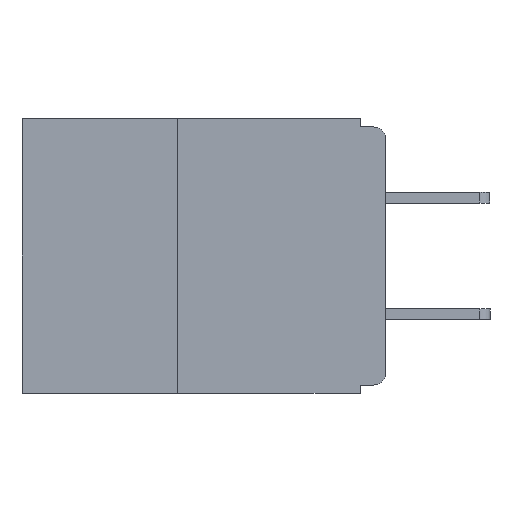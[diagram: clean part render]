
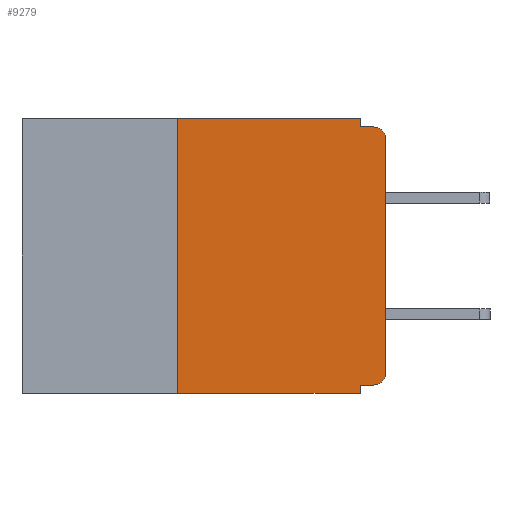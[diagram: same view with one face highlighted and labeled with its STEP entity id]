
A CAD part, left-side view. The second image highlights one B-rep face of the part: STEP entity #9279.
In plain terms, the highlighted planar face has unit normal (-1, 0, 0).
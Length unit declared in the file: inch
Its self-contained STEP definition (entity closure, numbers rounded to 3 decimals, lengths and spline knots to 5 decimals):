
#222 = CARTESIAN_POINT ( 'NONE',  ( 0., 0.25, -0.33 ) ) ;
#572 = DIRECTION ( 'NONE',  ( 0., -1., 0. ) ) ;
#774 = CARTESIAN_POINT ( 'NONE',  ( 0., 0., -0.01 ) ) ;
#980 = VECTOR ( 'NONE', #4086, 39.37008 ) ;
#1192 = DIRECTION ( 'NONE',  ( 0., 1., 0. ) ) ;
#1337 = LINE ( 'NONE', #5362, #1765 ) ;
#1546 = AXIS2_PLACEMENT_3D ( 'NONE', #6348, #11543, #3697 ) ;
#1620 = AXIS2_PLACEMENT_3D ( 'NONE', #16402, #16381, #16363 ) ;
#1765 = VECTOR ( 'NONE', #13138, 39.37008 ) ;
#1864 = DIRECTION ( 'NONE',  ( -1., 0., 0. ) ) ;
#1917 = CARTESIAN_POINT ( 'NONE',  ( 0., 0.25, 0. ) ) ;
#2356 = EDGE_CURVE ( 'NONE', #12118, #11571, #12422, .T. ) ;
#2382 = VECTOR ( 'NONE', #11886, 39.37008 ) ;
#2617 = VERTEX_POINT ( 'NONE', #5564 ) ;
#3012 = EDGE_CURVE ( 'NONE', #12989, #3067, #9993, .T. ) ;
#3044 = VECTOR ( 'NONE', #572, 39.37008 ) ;
#3067 = VERTEX_POINT ( 'NONE', #11272 ) ;
#3249 = CARTESIAN_POINT ( 'NONE',  ( 0., 0.25, -0.33 ) ) ;
#3310 = ORIENTED_EDGE ( 'NONE', *, *, #14291, .T. ) ;
#3428 = DIRECTION ( 'NONE',  ( 0., 0., 1. ) ) ;
#3697 = DIRECTION ( 'NONE',  ( 0., 0., -1. ) ) ;
#3735 = ORIENTED_EDGE ( 'NONE', *, *, #9853, .T. ) ;
#3780 = ORIENTED_EDGE ( 'NONE', *, *, #7662, .F. ) ;
#3961 = ORIENTED_EDGE ( 'NONE', *, *, #3012, .T. ) ;
#3988 = DIRECTION ( 'NONE',  ( 0., 0., -1. ) ) ;
#4086 = DIRECTION ( 'NONE',  ( 0., 0., -1. ) ) ;
#4179 = ORIENTED_EDGE ( 'NONE', *, *, #16122, .F. ) ;
#5362 = CARTESIAN_POINT ( 'NONE',  ( 0., 0.437, 0. ) ) ;
#5399 = CARTESIAN_POINT ( 'NONE',  ( 0., 0.015, -0.32 ) ) ;
#5564 = CARTESIAN_POINT ( 'NONE',  ( 0., 0.031, 0. ) ) ;
#6177 = EDGE_CURVE ( 'NONE', #16425, #6324, #16328, .T. ) ;
#6249 = EDGE_CURVE ( 'NONE', #6316, #6324, #11846, .T. ) ;
#6273 = CARTESIAN_POINT ( 'NONE',  ( 0., 0.031, -0.32 ) ) ;
#6316 = VERTEX_POINT ( 'NONE', #15924 ) ;
#6324 = VERTEX_POINT ( 'NONE', #15846 ) ;
#6348 = CARTESIAN_POINT ( 'NONE',  ( 0., 0.437, 0. ) ) ;
#6741 = CARTESIAN_POINT ( 'NONE',  ( 0., 0.031, 0. ) ) ;
#7026 = VECTOR ( 'NONE', #1192, 39.37008 ) ;
#7049 = LINE ( 'NONE', #11306, #16777 ) ;
#7131 = VECTOR ( 'NONE', #3428, 39.37008 ) ;
#7381 = DIRECTION ( 'NONE',  ( 0., -1., 0. ) ) ;
#7662 = EDGE_CURVE ( 'NONE', #13566, #9763, #13954, .T. ) ;
#7985 = CARTESIAN_POINT ( 'NONE',  ( 0., 0., 0. ) ) ;
#8919 = PLANE ( 'NONE',  #1546 ) ;
#9279 = ADVANCED_FACE ( 'NONE', ( #13320 ), #8919, .F. ) ;
#9763 = VERTEX_POINT ( 'NONE', #1917 ) ;
#9853 = EDGE_CURVE ( 'NONE', #13566, #11571, #7049, .T. ) ;
#9993 = CIRCLE ( 'NONE', #15067, 0.015 ) ;
#10115 = ORIENTED_EDGE ( 'NONE', *, *, #14780, .F. ) ;
#10314 = ORIENTED_EDGE ( 'NONE', *, *, #6177, .F. ) ;
#10717 = EDGE_CURVE ( 'NONE', #2617, #16425, #11516, .T. ) ;
#11117 = ORIENTED_EDGE ( 'NONE', *, *, #10717, .F. ) ;
#11272 = CARTESIAN_POINT ( 'NONE',  ( 0., 0., -0.305 ) ) ;
#11306 = CARTESIAN_POINT ( 'NONE',  ( 0., 0.437, -0.33 ) ) ;
#11322 = VECTOR ( 'NONE', #14431, 39.37008 ) ;
#11516 = LINE ( 'NONE', #6741, #980 ) ;
#11543 = DIRECTION ( 'NONE',  ( 1., 0., 0. ) ) ;
#11571 = VERTEX_POINT ( 'NONE', #16553 ) ;
#11846 = CIRCLE ( 'NONE', #1620, 0.015 ) ;
#11886 = DIRECTION ( 'NONE',  ( 0., 0., -1. ) ) ;
#12118 = VERTEX_POINT ( 'NONE', #6273 ) ;
#12422 = LINE ( 'NONE', #14348, #2382 ) ;
#12748 = CARTESIAN_POINT ( 'NONE',  ( 0., 0.031, -0.01 ) ) ;
#12855 = CARTESIAN_POINT ( 'NONE',  ( 0., 0.015, -0.305 ) ) ;
#12989 = VERTEX_POINT ( 'NONE', #5399 ) ;
#13138 = DIRECTION ( 'NONE',  ( 0., -1., 0. ) ) ;
#13320 = FACE_OUTER_BOUND ( 'NONE', #15656, .T. ) ;
#13502 = ORIENTED_EDGE ( 'NONE', *, *, #2356, .F. ) ;
#13566 = VERTEX_POINT ( 'NONE', #222 ) ;
#13860 = LINE ( 'NONE', #16680, #7026 ) ;
#13954 = LINE ( 'NONE', #3249, #7131 ) ;
#14291 = EDGE_CURVE ( 'NONE', #3067, #6316, #15413, .T. ) ;
#14348 = CARTESIAN_POINT ( 'NONE',  ( 0., 0.031, -0.33 ) ) ;
#14431 = DIRECTION ( 'NONE',  ( 0., 0., 1. ) ) ;
#14780 = EDGE_CURVE ( 'NONE', #12989, #12118, #13860, .T. ) ;
#15067 = AXIS2_PLACEMENT_3D ( 'NONE', #12855, #1864, #3988 ) ;
#15413 = LINE ( 'NONE', #7985, #11322 ) ;
#15656 = EDGE_LOOP ( 'NONE', ( #3310, #15996, #10314, #11117, #4179, #3780, #3735, #13502, #10115, #3961 ) ) ;
#15846 = CARTESIAN_POINT ( 'NONE',  ( 0., 0.015, -0.01 ) ) ;
#15924 = CARTESIAN_POINT ( 'NONE',  ( 0., 0., -0.025 ) ) ;
#15996 = ORIENTED_EDGE ( 'NONE', *, *, #6249, .T. ) ;
#16122 = EDGE_CURVE ( 'NONE', #9763, #2617, #1337, .T. ) ;
#16328 = LINE ( 'NONE', #774, #3044 ) ;
#16363 = DIRECTION ( 'NONE',  ( 0., 0., -1. ) ) ;
#16381 = DIRECTION ( 'NONE',  ( -1., 0., 0. ) ) ;
#16402 = CARTESIAN_POINT ( 'NONE',  ( 0., 0.015, -0.025 ) ) ;
#16425 = VERTEX_POINT ( 'NONE', #12748 ) ;
#16553 = CARTESIAN_POINT ( 'NONE',  ( 0., 0.031, -0.33 ) ) ;
#16680 = CARTESIAN_POINT ( 'NONE',  ( 0., 0., -0.32 ) ) ;
#16777 = VECTOR ( 'NONE', #7381, 39.37008 ) ;
